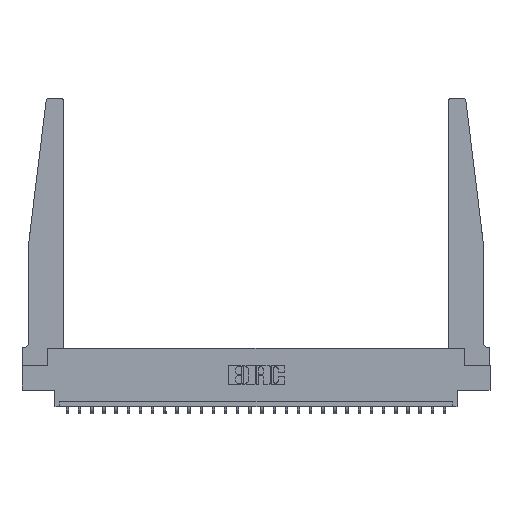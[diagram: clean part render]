
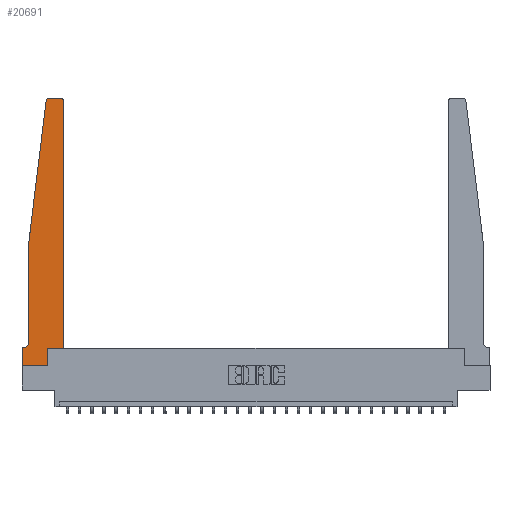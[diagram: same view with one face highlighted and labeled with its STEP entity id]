
A CAD part, top view. The second image highlights one B-rep face of the part: STEP entity #20691.
In plain terms, the highlighted planar face has unit normal (0, 0, 1).
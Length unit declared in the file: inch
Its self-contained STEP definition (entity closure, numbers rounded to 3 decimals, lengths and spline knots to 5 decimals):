
#54 = CARTESIAN_POINT ( 'NONE',  ( 0., 0., 0.37 ) ) ;
#69 = LINE ( 'NONE', #19974, #15600 ) ;
#161 = ORIENTED_EDGE ( 'NONE', *, *, #16348, .T. ) ;
#425 = EDGE_CURVE ( 'NONE', #10363, #14318, #7325, .T. ) ;
#488 = DIRECTION ( 'NONE',  ( 0., 0., 1. ) ) ;
#818 = ORIENTED_EDGE ( 'NONE', *, *, #15394, .T. ) ;
#1069 = ORIENTED_EDGE ( 'NONE', *, *, #425, .T. ) ;
#1118 = ORIENTED_EDGE ( 'NONE', *, *, #13528, .T. ) ;
#1195 = DIRECTION ( 'NONE',  ( 0., 1., 0. ) ) ;
#1406 = ORIENTED_EDGE ( 'NONE', *, *, #4916, .T. ) ;
#1432 = ORIENTED_EDGE ( 'NONE', *, *, #19387, .T. ) ;
#1707 = VECTOR ( 'NONE', #18658, 39.37008 ) ;
#1901 = LINE ( 'NONE', #25389, #16733 ) ;
#2004 = ORIENTED_EDGE ( 'NONE', *, *, #18674, .T. ) ;
#2293 = CARTESIAN_POINT ( 'NONE',  ( 0.395, 2.72, 0.37 ) ) ;
#2304 = CARTESIAN_POINT ( 'NONE',  ( 0.065, 0.2375, 0.37 ) ) ;
#2347 = VERTEX_POINT ( 'NONE', #16874 ) ;
#2425 = ORIENTED_EDGE ( 'NONE', *, *, #11510, .T. ) ;
#2763 = ORIENTED_EDGE ( 'NONE', *, *, #24325, .T. ) ;
#2767 = ORIENTED_EDGE ( 'NONE', *, *, #12912, .T. ) ;
#4058 = CARTESIAN_POINT ( 'NONE',  ( 0.425, 0.18, 0.37 ) ) ;
#4223 = DIRECTION ( 'NONE',  ( -0.122, -0.992, 0. ) ) ;
#4370 = DIRECTION ( 'NONE',  ( 1., 0., 0. ) ) ;
#4639 = VERTEX_POINT ( 'NONE', #23417 ) ;
#4670 = CARTESIAN_POINT ( 'NONE',  ( 0.015, 0.2375, 0.37 ) ) ;
#4916 = EDGE_CURVE ( 'NONE', #20714, #17537, #17159, .T. ) ;
#5713 = VECTOR ( 'NONE', #16005, 39.37008 ) ;
#6001 = CARTESIAN_POINT ( 'NONE',  ( 0., 0.1875, 0.37 ) ) ;
#6249 = CARTESIAN_POINT ( 'NONE',  ( 0.2605, 0.18, 0.37 ) ) ;
#6457 = CARTESIAN_POINT ( 'NONE',  ( 0.395, 2.75, 0.37 ) ) ;
#6722 = DIRECTION ( 'NONE',  ( -1., 0., 0. ) ) ;
#7325 = CIRCLE ( 'NONE', #17187, 0.05 ) ;
#7778 = AXIS2_PLACEMENT_3D ( 'NONE', #11932, #24027, #12022 ) ;
#8217 = DIRECTION ( 'NONE',  ( 0., -1., 0. ) ) ;
#9150 = ORIENTED_EDGE ( 'NONE', *, *, #19682, .T. ) ;
#9700 = VECTOR ( 'NONE', #23295, 39.37008 ) ;
#9989 = PLANE ( 'NONE',  #7778 ) ;
#10321 = ORIENTED_EDGE ( 'NONE', *, *, #11195, .T. ) ;
#10363 = VERTEX_POINT ( 'NONE', #2304 ) ;
#11188 = CARTESIAN_POINT ( 'NONE',  ( 0.065, 1.25, 0.37 ) ) ;
#11195 = EDGE_CURVE ( 'NONE', #14667, #11992, #12551, .T. ) ;
#11510 = EDGE_CURVE ( 'NONE', #25020, #24582, #69, .T. ) ;
#11735 = VERTEX_POINT ( 'NONE', #12676 ) ;
#11932 = CARTESIAN_POINT ( 'NONE',  ( 0., 0.1875, 0.37 ) ) ;
#11992 = VERTEX_POINT ( 'NONE', #21393 ) ;
#12022 = DIRECTION ( 'NONE',  ( 1., 0., 0. ) ) ;
#12551 = LINE ( 'NONE', #14674, #1707 ) ;
#12588 = AXIS2_PLACEMENT_3D ( 'NONE', #2293, #16405, #4370 ) ;
#12676 = CARTESIAN_POINT ( 'NONE',  ( 0.065, 1.25, 0.37 ) ) ;
#12697 = CARTESIAN_POINT ( 'NONE',  ( 0.27653, 2.72, 0.37 ) ) ;
#12765 = LINE ( 'NONE', #14319, #16768 ) ;
#12912 = EDGE_CURVE ( 'NONE', #2347, #14667, #21503, .T. ) ;
#13528 = EDGE_CURVE ( 'NONE', #14318, #20714, #12765, .T. ) ;
#13632 = EDGE_LOOP ( 'NONE', ( #10321, #9150, #161, #818, #1069, #1118, #1406, #1432, #2004, #2425, #2763, #2767 ) ) ;
#14073 = LINE ( 'NONE', #4058, #23462 ) ;
#14188 = FACE_OUTER_BOUND ( 'NONE', #13632, .T. ) ;
#14318 = VERTEX_POINT ( 'NONE', #15093 ) ;
#14319 = CARTESIAN_POINT ( 'NONE',  ( 0.065, 0.1875, 0.37 ) ) ;
#14667 = VERTEX_POINT ( 'NONE', #6457 ) ;
#14674 = CARTESIAN_POINT ( 'NONE',  ( 0.25, 2.75, 0.37 ) ) ;
#14676 = DIRECTION ( 'NONE',  ( 1., 0., 0. ) ) ;
#14969 = LINE ( 'NONE', #18266, #20273 ) ;
#15093 = CARTESIAN_POINT ( 'NONE',  ( 0.015, 0.1875, 0.37 ) ) ;
#15394 = EDGE_CURVE ( 'NONE', #11735, #10363, #20974, .T. ) ;
#15600 = VECTOR ( 'NONE', #18043, 39.37008 ) ;
#16000 = AXIS2_PLACEMENT_3D ( 'NONE', #12697, #488, #14676 ) ;
#16005 = DIRECTION ( 'NONE',  ( 1., 0., 0. ) ) ;
#16287 = DIRECTION ( 'NONE',  ( -1., 0., 0. ) ) ;
#16348 = EDGE_CURVE ( 'NONE', #4639, #11735, #14969, .T. ) ;
#16405 = DIRECTION ( 'NONE',  ( 0., 0., 1. ) ) ;
#16733 = VECTOR ( 'NONE', #1195, 39.37008 ) ;
#16768 = VECTOR ( 'NONE', #16287, 39.37008 ) ;
#16874 = CARTESIAN_POINT ( 'NONE',  ( 0.425, 2.72, 0.37 ) ) ;
#17159 = LINE ( 'NONE', #54, #21915 ) ;
#17187 = AXIS2_PLACEMENT_3D ( 'NONE', #4670, #18706, #6722 ) ;
#17537 = VERTEX_POINT ( 'NONE', #22103 ) ;
#18043 = DIRECTION ( 'NONE',  ( 1., 0., 0. ) ) ;
#18046 = VERTEX_POINT ( 'NONE', #21441 ) ;
#18266 = CARTESIAN_POINT ( 'NONE',  ( 0.065, 1.25, 0.37 ) ) ;
#18658 = DIRECTION ( 'NONE',  ( -1., 0., 0. ) ) ;
#18674 = EDGE_CURVE ( 'NONE', #18046, #25020, #1901, .T. ) ;
#18706 = DIRECTION ( 'NONE',  ( 0., 0., -1. ) ) ;
#19387 = EDGE_CURVE ( 'NONE', #17537, #18046, #22394, .T. ) ;
#19682 = EDGE_CURVE ( 'NONE', #11992, #4639, #25521, .T. ) ;
#19930 = CARTESIAN_POINT ( 'NONE',  ( 0., 0., 0.37 ) ) ;
#19974 = CARTESIAN_POINT ( 'NONE',  ( 0.425, 0.18, 0.37 ) ) ;
#20126 = DIRECTION ( 'NONE',  ( 0., 1., 0. ) ) ;
#20273 = VECTOR ( 'NONE', #4223, 39.37008 ) ;
#20691 = ADVANCED_FACE ( 'NONE', ( #14188 ), #9989, .T. ) ;
#20714 = VERTEX_POINT ( 'NONE', #6001 ) ;
#20911 = CARTESIAN_POINT ( 'NONE',  ( 0.425, 0.18, 0.37 ) ) ;
#20974 = LINE ( 'NONE', #11188, #9700 ) ;
#21393 = CARTESIAN_POINT ( 'NONE',  ( 0.27653, 2.75, 0.37 ) ) ;
#21441 = CARTESIAN_POINT ( 'NONE',  ( 0.2605, 0., 0.37 ) ) ;
#21503 = CIRCLE ( 'NONE', #12588, 0.03 ) ;
#21915 = VECTOR ( 'NONE', #8217, 39.37008 ) ;
#22103 = CARTESIAN_POINT ( 'NONE',  ( 0., 0., 0.37 ) ) ;
#22394 = LINE ( 'NONE', #19930, #5713 ) ;
#23295 = DIRECTION ( 'NONE',  ( 0., -1., 0. ) ) ;
#23417 = CARTESIAN_POINT ( 'NONE',  ( 0.24675, 2.72367, 0.37 ) ) ;
#23462 = VECTOR ( 'NONE', #20126, 39.37008 ) ;
#24027 = DIRECTION ( 'NONE',  ( 0., 0., 1. ) ) ;
#24325 = EDGE_CURVE ( 'NONE', #24582, #2347, #14073, .T. ) ;
#24582 = VERTEX_POINT ( 'NONE', #20911 ) ;
#25020 = VERTEX_POINT ( 'NONE', #6249 ) ;
#25389 = CARTESIAN_POINT ( 'NONE',  ( 0.2605, 0.18, 0.37 ) ) ;
#25521 = CIRCLE ( 'NONE', #16000, 0.03 ) ;
